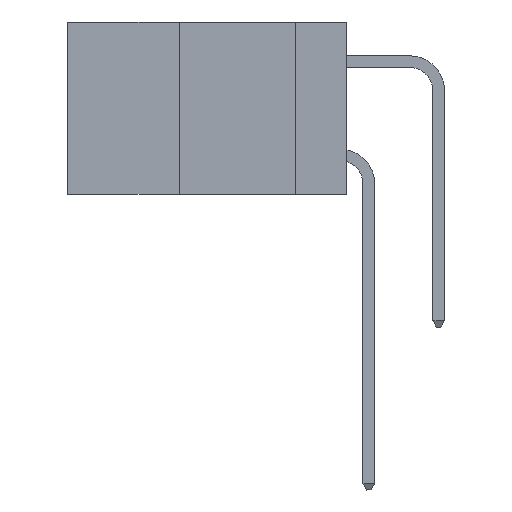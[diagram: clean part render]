
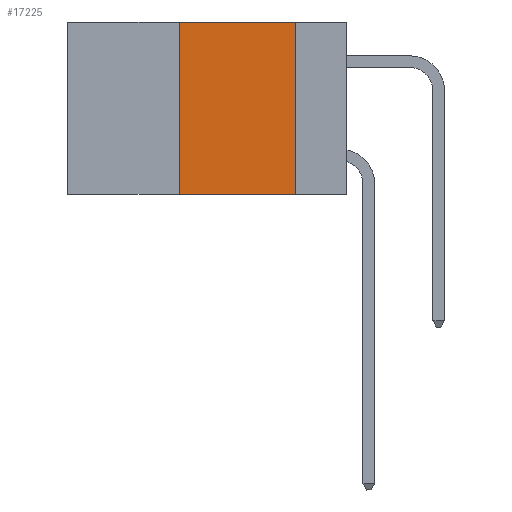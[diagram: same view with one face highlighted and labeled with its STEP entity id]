
A CAD part, left-side view. The second image highlights one B-rep face of the part: STEP entity #17225.
In plain terms, the highlighted planar face has unit normal (-1, 0, 0).
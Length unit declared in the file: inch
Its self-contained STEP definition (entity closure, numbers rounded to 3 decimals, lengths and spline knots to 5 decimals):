
#275 = DIRECTION ( 'NONE',  ( 0., 0., 1. ) ) ;
#1388 = ORIENTED_EDGE ( 'NONE', *, *, #25312, .F. ) ;
#1786 = CARTESIAN_POINT ( 'NONE',  ( 0., 0.36, 0. ) ) ;
#2469 = DIRECTION ( 'NONE',  ( 0., -1., 0. ) ) ;
#4112 = PLANE ( 'NONE',  #18463 ) ;
#4998 = CARTESIAN_POINT ( 'NONE',  ( 0., 0.6, -0.37 ) ) ;
#5154 = ORIENTED_EDGE ( 'NONE', *, *, #21679, .T. ) ;
#5199 = LINE ( 'NONE', #21745, #23996 ) ;
#5516 = LINE ( 'NONE', #23436, #27363 ) ;
#5886 = LINE ( 'NONE', #13549, #18828 ) ;
#6345 = DIRECTION ( 'NONE',  ( 1., 0., 0. ) ) ;
#7367 = EDGE_LOOP ( 'NONE', ( #1388, #14093, #12587, #5154 ) ) ;
#7828 = EDGE_CURVE ( 'NONE', #10159, #10177, #5199, .T. ) ;
#8265 = CARTESIAN_POINT ( 'NONE',  ( 0., 0.36, -0.37 ) ) ;
#10159 = VERTEX_POINT ( 'NONE', #1786 ) ;
#10177 = VERTEX_POINT ( 'NONE', #23543 ) ;
#10403 = DIRECTION ( 'NONE',  ( 0., 0., -1. ) ) ;
#12587 = ORIENTED_EDGE ( 'NONE', *, *, #17847, .F. ) ;
#13549 = CARTESIAN_POINT ( 'NONE',  ( 0., 0.36, 0. ) ) ;
#14093 = ORIENTED_EDGE ( 'NONE', *, *, #7828, .F. ) ;
#17225 = ADVANCED_FACE ( 'NONE', ( #27412 ), #4112, .F. ) ;
#17847 = EDGE_CURVE ( 'NONE', #20516, #10159, #5886, .T. ) ;
#18463 = AXIS2_PLACEMENT_3D ( 'NONE', #19360, #6345, #23782 ) ;
#18828 = VECTOR ( 'NONE', #275, 39.37008 ) ;
#19360 = CARTESIAN_POINT ( 'NONE',  ( 0., 0.6, 0. ) ) ;
#20089 = DIRECTION ( 'NONE',  ( 0., -1., 0. ) ) ;
#20516 = VERTEX_POINT ( 'NONE', #8265 ) ;
#20800 = VERTEX_POINT ( 'NONE', #27961 ) ;
#21679 = EDGE_CURVE ( 'NONE', #20516, #20800, #23833, .T. ) ;
#21745 = CARTESIAN_POINT ( 'NONE',  ( 0., 0.6, 0. ) ) ;
#23436 = CARTESIAN_POINT ( 'NONE',  ( 0., 0.11, 0. ) ) ;
#23543 = CARTESIAN_POINT ( 'NONE',  ( 0., 0.11, 0. ) ) ;
#23782 = DIRECTION ( 'NONE',  ( 0., 0., -1. ) ) ;
#23833 = LINE ( 'NONE', #4998, #27933 ) ;
#23996 = VECTOR ( 'NONE', #2469, 39.37008 ) ;
#25312 = EDGE_CURVE ( 'NONE', #10177, #20800, #5516, .T. ) ;
#27363 = VECTOR ( 'NONE', #10403, 39.37008 ) ;
#27412 = FACE_OUTER_BOUND ( 'NONE', #7367, .T. ) ;
#27933 = VECTOR ( 'NONE', #20089, 39.37008 ) ;
#27961 = CARTESIAN_POINT ( 'NONE',  ( 0., 0.11, -0.37 ) ) ;
